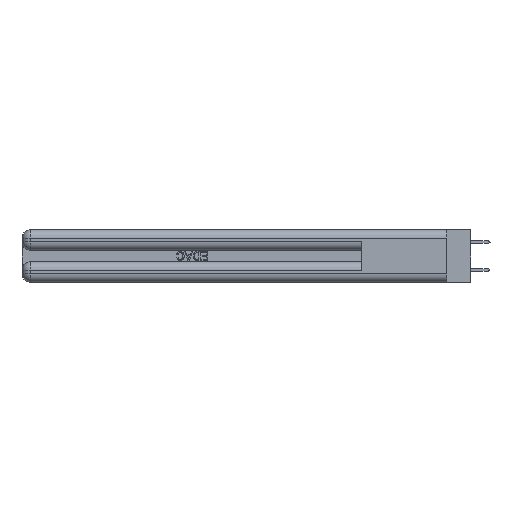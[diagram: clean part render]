
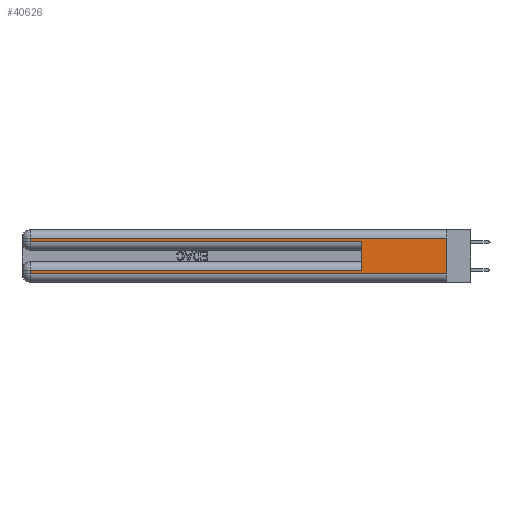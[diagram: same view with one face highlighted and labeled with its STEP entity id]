
A CAD part, left-side view. The second image highlights one B-rep face of the part: STEP entity #40626.
In plain terms, the highlighted planar face has unit normal (-1, 0, 0).
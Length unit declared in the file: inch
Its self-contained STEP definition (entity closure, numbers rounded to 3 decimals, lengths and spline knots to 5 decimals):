
#254 = CARTESIAN_POINT ( 'NONE',  ( 0., 2.94, 0.085 ) ) ;
#318 = ORIENTED_EDGE ( 'NONE', *, *, #26221, .T. ) ;
#638 = EDGE_CURVE ( 'NONE', #3155, #22956, #22386, .T. ) ;
#797 = ORIENTED_EDGE ( 'NONE', *, *, #17920, .T. ) ;
#836 = LINE ( 'NONE', #3673, #12315 ) ;
#1273 = CARTESIAN_POINT ( 'NONE',  ( 0., 0.6, 0.145 ) ) ;
#1473 = CARTESIAN_POINT ( 'NONE',  ( 0., 2.94, 0.06 ) ) ;
#3155 = VERTEX_POINT ( 'NONE', #6838 ) ;
#3453 = LINE ( 'NONE', #24341, #36858 ) ;
#3673 = CARTESIAN_POINT ( 'NONE',  ( 0., 0., 0.085 ) ) ;
#3712 = ORIENTED_EDGE ( 'NONE', *, *, #12935, .T. ) ;
#3979 = VECTOR ( 'NONE', #29535, 39.37008 ) ;
#4772 = VECTOR ( 'NONE', #18336, 39.37008 ) ;
#6041 = EDGE_CURVE ( 'NONE', #9056, #20153, #41552, .T. ) ;
#6735 = CARTESIAN_POINT ( 'NONE',  ( 0., 0., 0.06 ) ) ;
#6787 = VERTEX_POINT ( 'NONE', #27168 ) ;
#6838 = CARTESIAN_POINT ( 'NONE',  ( 0., 0.6, 0.085 ) ) ;
#9056 = VERTEX_POINT ( 'NONE', #1473 ) ;
#9101 = DIRECTION ( 'NONE',  ( 0., -1., 0. ) ) ;
#10052 = DIRECTION ( 'NONE',  ( 0., 0., -1. ) ) ;
#10761 = LINE ( 'NONE', #25682, #4772 ) ;
#11514 = LINE ( 'NONE', #14368, #3979 ) ;
#12315 = VECTOR ( 'NONE', #21945, 39.37008 ) ;
#12860 = EDGE_CURVE ( 'NONE', #3155, #26689, #836, .T. ) ;
#12935 = EDGE_CURVE ( 'NONE', #42465, #16125, #11514, .T. ) ;
#13347 = EDGE_CURVE ( 'NONE', #6787, #20153, #10761, .T. ) ;
#14368 = CARTESIAN_POINT ( 'NONE',  ( 0., 2.94, 0.37 ) ) ;
#14935 = CARTESIAN_POINT ( 'NONE',  ( 0., 2.94, 0.285 ) ) ;
#15747 = DIRECTION ( 'NONE',  ( 0., 0., 1. ) ) ;
#16125 = VERTEX_POINT ( 'NONE', #14935 ) ;
#16210 = CARTESIAN_POINT ( 'NONE',  ( 0., 2.94, 0.31 ) ) ;
#16311 = VECTOR ( 'NONE', #36914, 39.37008 ) ;
#17567 = ORIENTED_EDGE ( 'NONE', *, *, #638, .F. ) ;
#17920 = EDGE_CURVE ( 'NONE', #26689, #9056, #29579, .T. ) ;
#18336 = DIRECTION ( 'NONE',  ( 0., 0., -1. ) ) ;
#20153 = VERTEX_POINT ( 'NONE', #6735 ) ;
#20563 = ORIENTED_EDGE ( 'NONE', *, *, #30953, .T. ) ;
#20704 = CARTESIAN_POINT ( 'NONE',  ( 0., 0., 0.06 ) ) ;
#20980 = DIRECTION ( 'NONE',  ( 0., 1., 0. ) ) ;
#21945 = DIRECTION ( 'NONE',  ( 0., 1., 0. ) ) ;
#22386 = LINE ( 'NONE', #1273, #37211 ) ;
#22460 = CARTESIAN_POINT ( 'NONE',  ( 0., 2.94, 0.37 ) ) ;
#22956 = VERTEX_POINT ( 'NONE', #33836 ) ;
#24341 = CARTESIAN_POINT ( 'NONE',  ( 0., 0., 0.285 ) ) ;
#24571 = ORIENTED_EDGE ( 'NONE', *, *, #6041, .T. ) ;
#24798 = DIRECTION ( 'NONE',  ( 0., -1., 0. ) ) ;
#25482 = LINE ( 'NONE', #42764, #40901 ) ;
#25682 = CARTESIAN_POINT ( 'NONE',  ( 0., 0., 0.37 ) ) ;
#26171 = ORIENTED_EDGE ( 'NONE', *, *, #13347, .F. ) ;
#26221 = EDGE_CURVE ( 'NONE', #16125, #22956, #3453, .T. ) ;
#26689 = VERTEX_POINT ( 'NONE', #254 ) ;
#27131 = PLANE ( 'NONE',  #43282 ) ;
#27168 = CARTESIAN_POINT ( 'NONE',  ( 0., 0., 0.31 ) ) ;
#27604 = FACE_OUTER_BOUND ( 'NONE', #43116, .T. ) ;
#29535 = DIRECTION ( 'NONE',  ( 0., 0., -1. ) ) ;
#29579 = LINE ( 'NONE', #22460, #16311 ) ;
#30953 = EDGE_CURVE ( 'NONE', #6787, #42465, #25482, .T. ) ;
#33836 = CARTESIAN_POINT ( 'NONE',  ( 0., 0.6, 0.285 ) ) ;
#34949 = DIRECTION ( 'NONE',  ( 1., 0., 0. ) ) ;
#35847 = ORIENTED_EDGE ( 'NONE', *, *, #12860, .T. ) ;
#36858 = VECTOR ( 'NONE', #24798, 39.37008 ) ;
#36914 = DIRECTION ( 'NONE',  ( 0., 0., -1. ) ) ;
#37211 = VECTOR ( 'NONE', #15747, 39.37008 ) ;
#40626 = ADVANCED_FACE ( 'NONE', ( #27604 ), #27131, .F. ) ;
#40901 = VECTOR ( 'NONE', #20980, 39.37008 ) ;
#41552 = LINE ( 'NONE', #20704, #45330 ) ;
#41815 = CARTESIAN_POINT ( 'NONE',  ( 0., 0., 0.37 ) ) ;
#42465 = VERTEX_POINT ( 'NONE', #16210 ) ;
#42764 = CARTESIAN_POINT ( 'NONE',  ( 0., 0., 0.31 ) ) ;
#43116 = EDGE_LOOP ( 'NONE', ( #26171, #20563, #3712, #318, #17567, #35847, #797, #24571 ) ) ;
#43282 = AXIS2_PLACEMENT_3D ( 'NONE', #41815, #34949, #10052 ) ;
#45330 = VECTOR ( 'NONE', #9101, 39.37008 ) ;
